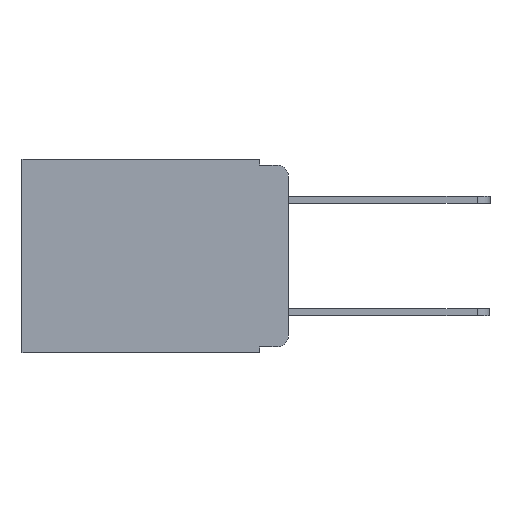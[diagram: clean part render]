
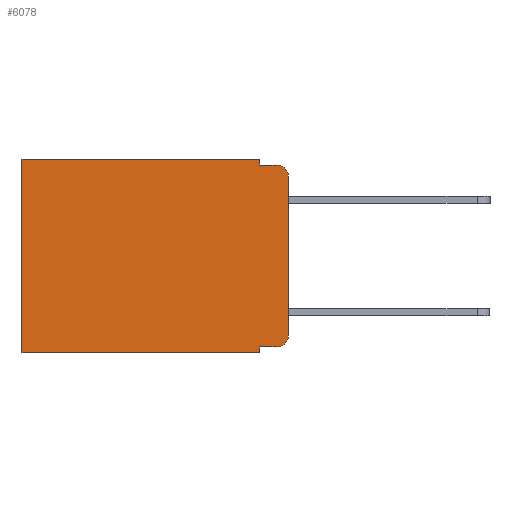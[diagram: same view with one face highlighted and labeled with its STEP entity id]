
A CAD part, left-side view. The second image highlights one B-rep face of the part: STEP entity #6078.
In plain terms, the highlighted planar face has unit normal (-1, 0, 0).
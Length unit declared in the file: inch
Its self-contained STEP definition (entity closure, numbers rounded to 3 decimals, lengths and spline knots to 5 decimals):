
#192 = LINE ( 'NONE', #12245, #6081 ) ;
#289 = DIRECTION ( 'NONE',  ( 0., -1., 0. ) ) ;
#630 = VECTOR ( 'NONE', #7981, 39.37008 ) ;
#643 = VERTEX_POINT ( 'NONE', #1444 ) ;
#692 = EDGE_CURVE ( 'NONE', #6374, #4117, #7521, .T. ) ;
#1030 = DIRECTION ( 'NONE',  ( 0., 0., -1. ) ) ;
#1082 = CARTESIAN_POINT ( 'NONE',  ( 0.298, 0.051, 0. ) ) ;
#1134 = EDGE_CURVE ( 'NONE', #7380, #1169, #11377, .T. ) ;
#1169 = VERTEX_POINT ( 'NONE', #9705 ) ;
#1418 = VERTEX_POINT ( 'NONE', #3920 ) ;
#1444 = CARTESIAN_POINT ( 'NONE',  ( 0.298, 0.02, -0.01 ) ) ;
#1450 = VERTEX_POINT ( 'NONE', #1613 ) ;
#1537 = ORIENTED_EDGE ( 'NONE', *, *, #8147, .F. ) ;
#1613 = CARTESIAN_POINT ( 'NONE',  ( 0.298, 0.051, -0.343 ) ) ;
#1789 = VECTOR ( 'NONE', #1030, 39.37008 ) ;
#2429 = CARTESIAN_POINT ( 'NONE',  ( 0.298, 0., 0. ) ) ;
#2477 = ORIENTED_EDGE ( 'NONE', *, *, #6537, .T. ) ;
#2635 = AXIS2_PLACEMENT_3D ( 'NONE', #10520, #5056, #11357 ) ;
#2785 = VERTEX_POINT ( 'NONE', #12032 ) ;
#3090 = EDGE_LOOP ( 'NONE', ( #6743, #5331, #10993, #4880, #4706, #2477, #9681, #1537, #12184, #11021 ) ) ;
#3348 = CARTESIAN_POINT ( 'NONE',  ( 0.298, 0., -0.313 ) ) ;
#3432 = CARTESIAN_POINT ( 'NONE',  ( 0.298, 0.051, -0.01 ) ) ;
#3512 = EDGE_CURVE ( 'NONE', #1418, #4342, #9763, .T. ) ;
#3619 = CARTESIAN_POINT ( 'NONE',  ( 0.298, 0., -0.343 ) ) ;
#3722 = DIRECTION ( 'NONE',  ( 0., 1., 0. ) ) ;
#3903 = EDGE_CURVE ( 'NONE', #1418, #7061, #9090, .T. ) ;
#3920 = CARTESIAN_POINT ( 'NONE',  ( 0.298, 0.051, 0. ) ) ;
#3929 = EDGE_CURVE ( 'NONE', #7061, #643, #192, .T. ) ;
#3947 = VECTOR ( 'NONE', #11604, 39.37008 ) ;
#4117 = VERTEX_POINT ( 'NONE', #3348 ) ;
#4205 = CARTESIAN_POINT ( 'NONE',  ( 0.298, 0., 0. ) ) ;
#4228 = CIRCLE ( 'NONE', #5949, 0.02 ) ;
#4342 = VERTEX_POINT ( 'NONE', #7733 ) ;
#4371 = EDGE_CURVE ( 'NONE', #1450, #2785, #10128, .T. ) ;
#4559 = CARTESIAN_POINT ( 'NONE',  ( 0.298, 0.051, -0.333 ) ) ;
#4706 = ORIENTED_EDGE ( 'NONE', *, *, #3512, .T. ) ;
#4836 = DIRECTION ( 'NONE',  ( 1., 0., 0. ) ) ;
#4837 = EDGE_CURVE ( 'NONE', #1169, #4117, #11166, .T. ) ;
#4880 = ORIENTED_EDGE ( 'NONE', *, *, #3903, .F. ) ;
#4907 = VECTOR ( 'NONE', #6184, 39.37008 ) ;
#4955 = LINE ( 'NONE', #5647, #1789 ) ;
#5056 = DIRECTION ( 'NONE',  ( -1., 0., 0. ) ) ;
#5331 = ORIENTED_EDGE ( 'NONE', *, *, #6670, .T. ) ;
#5563 = LINE ( 'NONE', #1082, #10113 ) ;
#5647 = CARTESIAN_POINT ( 'NONE',  ( 0.298, 0.473, 0. ) ) ;
#5921 = FACE_OUTER_BOUND ( 'NONE', #3090, .T. ) ;
#5949 = AXIS2_PLACEMENT_3D ( 'NONE', #12007, #6831, #12835 ) ;
#6078 = ADVANCED_FACE ( 'NONE', ( #5921 ), #6806, .F. ) ;
#6081 = VECTOR ( 'NONE', #289, 39.37008 ) ;
#6184 = DIRECTION ( 'NONE',  ( 0., 0., -1. ) ) ;
#6373 = CARTESIAN_POINT ( 'NONE',  ( 0.298, 0., -0.03 ) ) ;
#6374 = VERTEX_POINT ( 'NONE', #6373 ) ;
#6458 = AXIS2_PLACEMENT_3D ( 'NONE', #2429, #4836, #11171 ) ;
#6537 = EDGE_CURVE ( 'NONE', #4342, #2785, #4955, .T. ) ;
#6670 = EDGE_CURVE ( 'NONE', #6374, #643, #4228, .T. ) ;
#6743 = ORIENTED_EDGE ( 'NONE', *, *, #692, .F. ) ;
#6806 = PLANE ( 'NONE',  #6458 ) ;
#6831 = DIRECTION ( 'NONE',  ( -1., 0., 0. ) ) ;
#7061 = VERTEX_POINT ( 'NONE', #3432 ) ;
#7089 = CARTESIAN_POINT ( 'NONE',  ( 0.298, 0.051, 0. ) ) ;
#7380 = VERTEX_POINT ( 'NONE', #8840 ) ;
#7521 = LINE ( 'NONE', #4205, #4907 ) ;
#7568 = VECTOR ( 'NONE', #10339, 39.37008 ) ;
#7733 = CARTESIAN_POINT ( 'NONE',  ( 0.298, 0.473, 0. ) ) ;
#7809 = CARTESIAN_POINT ( 'NONE',  ( 0.298, 0., 0. ) ) ;
#7981 = DIRECTION ( 'NONE',  ( 0., 0., -1. ) ) ;
#8147 = EDGE_CURVE ( 'NONE', #7380, #1450, #5563, .T. ) ;
#8840 = CARTESIAN_POINT ( 'NONE',  ( 0.298, 0.051, -0.333 ) ) ;
#9090 = LINE ( 'NONE', #7089, #630 ) ;
#9391 = DIRECTION ( 'NONE',  ( 0., 0., -1. ) ) ;
#9681 = ORIENTED_EDGE ( 'NONE', *, *, #4371, .F. ) ;
#9705 = CARTESIAN_POINT ( 'NONE',  ( 0.298, 0.02, -0.333 ) ) ;
#9763 = LINE ( 'NONE', #7809, #12262 ) ;
#10113 = VECTOR ( 'NONE', #9391, 39.37008 ) ;
#10128 = LINE ( 'NONE', #3619, #7568 ) ;
#10339 = DIRECTION ( 'NONE',  ( 0., 1., 0. ) ) ;
#10520 = CARTESIAN_POINT ( 'NONE',  ( 0.298, 0.02, -0.313 ) ) ;
#10993 = ORIENTED_EDGE ( 'NONE', *, *, #3929, .F. ) ;
#11021 = ORIENTED_EDGE ( 'NONE', *, *, #4837, .T. ) ;
#11166 = CIRCLE ( 'NONE', #2635, 0.02 ) ;
#11171 = DIRECTION ( 'NONE',  ( 0., 0., -1. ) ) ;
#11357 = DIRECTION ( 'NONE',  ( 0., 0., -1. ) ) ;
#11377 = LINE ( 'NONE', #4559, #3947 ) ;
#11604 = DIRECTION ( 'NONE',  ( 0., -1., 0. ) ) ;
#12007 = CARTESIAN_POINT ( 'NONE',  ( 0.298, 0.02, -0.03 ) ) ;
#12032 = CARTESIAN_POINT ( 'NONE',  ( 0.298, 0.473, -0.343 ) ) ;
#12184 = ORIENTED_EDGE ( 'NONE', *, *, #1134, .T. ) ;
#12245 = CARTESIAN_POINT ( 'NONE',  ( 0.298, 0.051, -0.01 ) ) ;
#12262 = VECTOR ( 'NONE', #3722, 39.37008 ) ;
#12835 = DIRECTION ( 'NONE',  ( 0., 0., -1. ) ) ;
